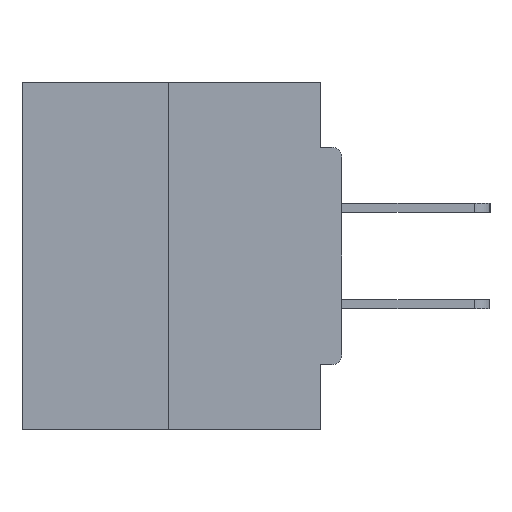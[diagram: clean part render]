
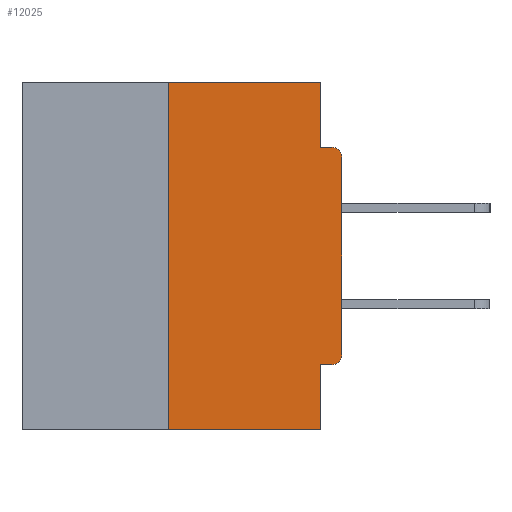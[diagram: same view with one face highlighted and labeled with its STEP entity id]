
A CAD part, left-side view. The second image highlights one B-rep face of the part: STEP entity #12025.
In plain terms, the highlighted planar face has unit normal (-1, 0, 0).
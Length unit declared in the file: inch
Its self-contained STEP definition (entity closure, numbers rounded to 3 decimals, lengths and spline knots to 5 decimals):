
#322 = CARTESIAN_POINT ( 'NONE',  ( 0., 0., -0.3915 ) ) ;
#969 = LINE ( 'NONE', #26049, #21778 ) ;
#1536 = VECTOR ( 'NONE', #4673, 39.37008 ) ;
#2036 = VERTEX_POINT ( 'NONE', #26186 ) ;
#2042 = VECTOR ( 'NONE', #22094, 39.37008 ) ;
#2229 = CARTESIAN_POINT ( 'NONE',  ( 0., 0.46, -0.5 ) ) ;
#2394 = VERTEX_POINT ( 'NONE', #21415 ) ;
#2419 = ORIENTED_EDGE ( 'NONE', *, *, #2885, .F. ) ;
#2885 = EDGE_CURVE ( 'NONE', #30506, #2394, #21544, .T. ) ;
#3255 = EDGE_CURVE ( 'NONE', #31228, #27552, #12981, .T. ) ;
#3779 = LINE ( 'NONE', #31254, #17703 ) ;
#3878 = AXIS2_PLACEMENT_3D ( 'NONE', #25030, #17803, #30615 ) ;
#4041 = ORIENTED_EDGE ( 'NONE', *, *, #6676, .F. ) ;
#4673 = DIRECTION ( 'NONE',  ( 0., 0., -1. ) ) ;
#5945 = CARTESIAN_POINT ( 'NONE',  ( 0., 0.031, 0. ) ) ;
#6460 = ORIENTED_EDGE ( 'NONE', *, *, #8734, .F. ) ;
#6676 = EDGE_CURVE ( 'NONE', #2036, #8704, #969, .T. ) ;
#6882 = CARTESIAN_POINT ( 'NONE',  ( 0., 0., -0.1085 ) ) ;
#7127 = EDGE_CURVE ( 'NONE', #31437, #31228, #18436, .T. ) ;
#7190 = LINE ( 'NONE', #17477, #1536 ) ;
#7330 = ORIENTED_EDGE ( 'NONE', *, *, #11538, .F. ) ;
#7524 = VECTOR ( 'NONE', #13122, 39.37008 ) ;
#7607 = VECTOR ( 'NONE', #16841, 39.37008 ) ;
#7713 = VERTEX_POINT ( 'NONE', #9739 ) ;
#7908 = LINE ( 'NONE', #18192, #7524 ) ;
#8365 = DIRECTION ( 'NONE',  ( 0., 1., 0. ) ) ;
#8704 = VERTEX_POINT ( 'NONE', #33231 ) ;
#8734 = EDGE_CURVE ( 'NONE', #2394, #27552, #31039, .T. ) ;
#9739 = CARTESIAN_POINT ( 'NONE',  ( 0., 0.25, 0. ) ) ;
#9866 = EDGE_CURVE ( 'NONE', #15180, #24261, #27487, .T. ) ;
#9880 = DIRECTION ( 'NONE',  ( 1., 0., 0. ) ) ;
#10276 = ORIENTED_EDGE ( 'NONE', *, *, #9866, .T. ) ;
#10294 = DIRECTION ( 'NONE',  ( 0., -1., 0. ) ) ;
#10716 = CARTESIAN_POINT ( 'NONE',  ( 0., 0.031, -0.5 ) ) ;
#11538 = EDGE_CURVE ( 'NONE', #7713, #30506, #3779, .T. ) ;
#11916 = AXIS2_PLACEMENT_3D ( 'NONE', #15787, #31922, #28421 ) ;
#12025 = ADVANCED_FACE ( 'NONE', ( #22838 ), #12401, .F. ) ;
#12162 = EDGE_CURVE ( 'NONE', #8704, #24261, #7190, .T. ) ;
#12233 = CARTESIAN_POINT ( 'NONE',  ( 0., 0.46, 0. ) ) ;
#12401 = PLANE ( 'NONE',  #25165 ) ;
#12813 = CARTESIAN_POINT ( 'NONE',  ( 0., 0., -0.0935 ) ) ;
#12981 = CIRCLE ( 'NONE', #11916, 0.015 ) ;
#13122 = DIRECTION ( 'NONE',  ( 0., 0., 1. ) ) ;
#13725 = VECTOR ( 'NONE', #26975, 39.37008 ) ;
#14098 = ORIENTED_EDGE ( 'NONE', *, *, #20840, .T. ) ;
#15180 = VERTEX_POINT ( 'NONE', #30943 ) ;
#15787 = CARTESIAN_POINT ( 'NONE',  ( 0., 0.015, -0.1085 ) ) ;
#16094 = EDGE_LOOP ( 'NONE', ( #7330, #22428, #10276, #21010, #4041, #14098, #30774, #18235, #6460, #2419 ) ) ;
#16551 = CARTESIAN_POINT ( 'NONE',  ( 0., 0., 0. ) ) ;
#16841 = DIRECTION ( 'NONE',  ( 0., 0., -1. ) ) ;
#16973 = EDGE_CURVE ( 'NONE', #15180, #7713, #7908, .T. ) ;
#16984 = DIRECTION ( 'NONE',  ( 0., 0., -1. ) ) ;
#17006 = CARTESIAN_POINT ( 'NONE',  ( 0., 0.031, 0. ) ) ;
#17295 = CARTESIAN_POINT ( 'NONE',  ( 0., 0.015, -0.0935 ) ) ;
#17477 = CARTESIAN_POINT ( 'NONE',  ( 0., 0.031, -0.5 ) ) ;
#17703 = VECTOR ( 'NONE', #29040, 39.37008 ) ;
#17803 = DIRECTION ( 'NONE',  ( -1., 0., 0. ) ) ;
#18192 = CARTESIAN_POINT ( 'NONE',  ( 0., 0.25, 0. ) ) ;
#18235 = ORIENTED_EDGE ( 'NONE', *, *, #3255, .T. ) ;
#18436 = LINE ( 'NONE', #16551, #13725 ) ;
#20840 = EDGE_CURVE ( 'NONE', #2036, #31437, #32931, .T. ) ;
#21010 = ORIENTED_EDGE ( 'NONE', *, *, #12162, .F. ) ;
#21415 = CARTESIAN_POINT ( 'NONE',  ( 0., 0.031, -0.0935 ) ) ;
#21544 = LINE ( 'NONE', #17006, #7607 ) ;
#21778 = VECTOR ( 'NONE', #8365, 39.37008 ) ;
#22094 = DIRECTION ( 'NONE',  ( 0., -1., 0. ) ) ;
#22428 = ORIENTED_EDGE ( 'NONE', *, *, #16973, .F. ) ;
#22838 = FACE_OUTER_BOUND ( 'NONE', #16094, .T. ) ;
#23482 = VECTOR ( 'NONE', #10294, 39.37008 ) ;
#24261 = VERTEX_POINT ( 'NONE', #10716 ) ;
#25030 = CARTESIAN_POINT ( 'NONE',  ( 0., 0.015, -0.3915 ) ) ;
#25165 = AXIS2_PLACEMENT_3D ( 'NONE', #12233, #9880, #16984 ) ;
#26049 = CARTESIAN_POINT ( 'NONE',  ( 0., 0., -0.4065 ) ) ;
#26186 = CARTESIAN_POINT ( 'NONE',  ( 0., 0.015, -0.4065 ) ) ;
#26975 = DIRECTION ( 'NONE',  ( 0., 0., 1. ) ) ;
#27487 = LINE ( 'NONE', #2229, #2042 ) ;
#27552 = VERTEX_POINT ( 'NONE', #17295 ) ;
#28421 = DIRECTION ( 'NONE',  ( 0., 0., -1. ) ) ;
#29040 = DIRECTION ( 'NONE',  ( 0., -1., 0. ) ) ;
#30506 = VERTEX_POINT ( 'NONE', #5945 ) ;
#30615 = DIRECTION ( 'NONE',  ( 0., 0., -1. ) ) ;
#30774 = ORIENTED_EDGE ( 'NONE', *, *, #7127, .T. ) ;
#30943 = CARTESIAN_POINT ( 'NONE',  ( 0., 0.25, -0.5 ) ) ;
#31039 = LINE ( 'NONE', #12813, #23482 ) ;
#31228 = VERTEX_POINT ( 'NONE', #6882 ) ;
#31254 = CARTESIAN_POINT ( 'NONE',  ( 0., 0.46, 0. ) ) ;
#31437 = VERTEX_POINT ( 'NONE', #322 ) ;
#31922 = DIRECTION ( 'NONE',  ( -1., 0., 0. ) ) ;
#32931 = CIRCLE ( 'NONE', #3878, 0.015 ) ;
#33231 = CARTESIAN_POINT ( 'NONE',  ( 0., 0.031, -0.4065 ) ) ;
